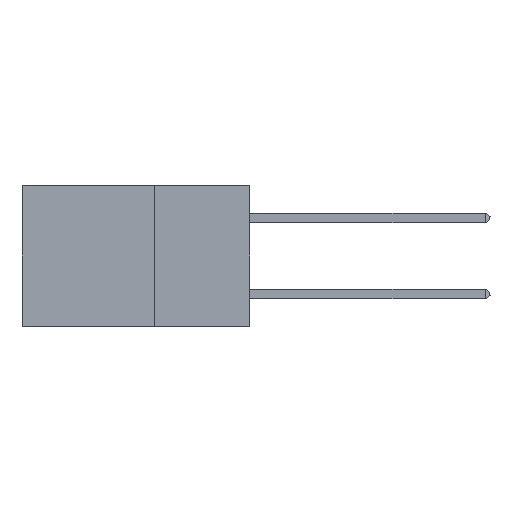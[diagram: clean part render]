
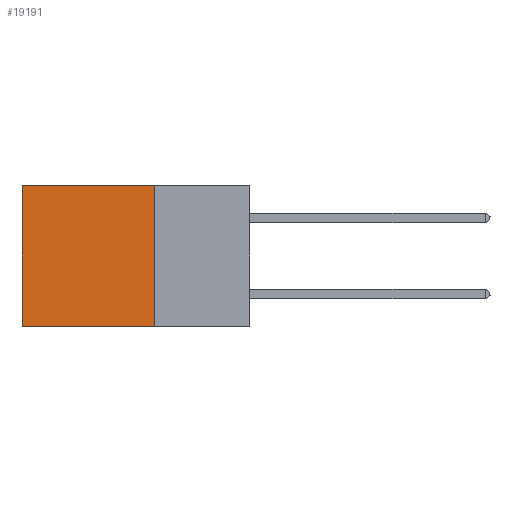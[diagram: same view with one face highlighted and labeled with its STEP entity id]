
A CAD part, left-side view. The second image highlights one B-rep face of the part: STEP entity #19191.
In plain terms, the highlighted planar face has unit normal (-1, 0, 0).
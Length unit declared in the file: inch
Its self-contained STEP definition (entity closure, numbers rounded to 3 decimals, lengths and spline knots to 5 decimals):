
#1883 = ORIENTED_EDGE ( 'NONE', *, *, #9768, .T. ) ;
#2938 = DIRECTION ( 'NONE',  ( 0., 1., 0. ) ) ;
#3231 = CARTESIAN_POINT ( 'NONE',  ( 0.2875, 0.25, -0.37 ) ) ;
#3572 = LINE ( 'NONE', #3231, #34149 ) ;
#4165 = LINE ( 'NONE', #35471, #8786 ) ;
#4431 = EDGE_LOOP ( 'NONE', ( #1883, #27763, #6067, #38843 ) ) ;
#4472 = CARTESIAN_POINT ( 'NONE',  ( 0.2875, 0.6, 0. ) ) ;
#6067 = ORIENTED_EDGE ( 'NONE', *, *, #7872, .F. ) ;
#7531 = LINE ( 'NONE', #43068, #9848 ) ;
#7872 = EDGE_CURVE ( 'NONE', #39668, #38257, #26251, .T. ) ;
#8786 = VECTOR ( 'NONE', #24356, 39.37008 ) ;
#9768 = EDGE_CURVE ( 'NONE', #15532, #27740, #4165, .T. ) ;
#9848 = VECTOR ( 'NONE', #2938, 39.37008 ) ;
#9864 = EDGE_CURVE ( 'NONE', #38257, #27740, #3572, .T. ) ;
#11196 = DIRECTION ( 'NONE',  ( 0., 0., -1. ) ) ;
#13850 = DIRECTION ( 'NONE',  ( 0., 1., 0. ) ) ;
#15532 = VERTEX_POINT ( 'NONE', #4472 ) ;
#15880 = CARTESIAN_POINT ( 'NONE',  ( 0.2875, 0.25, -0.37 ) ) ;
#19191 = ADVANCED_FACE ( 'NONE', ( #28418 ), #40385, .F. ) ;
#19772 = AXIS2_PLACEMENT_3D ( 'NONE', #40857, #47830, #11196 ) ;
#23465 = CARTESIAN_POINT ( 'NONE',  ( 0.2875, 0.25, 0. ) ) ;
#24356 = DIRECTION ( 'NONE',  ( 0., 0., -1. ) ) ;
#26251 = LINE ( 'NONE', #28870, #33779 ) ;
#27740 = VERTEX_POINT ( 'NONE', #31491 ) ;
#27763 = ORIENTED_EDGE ( 'NONE', *, *, #9864, .F. ) ;
#28418 = FACE_OUTER_BOUND ( 'NONE', #4431, .T. ) ;
#28870 = CARTESIAN_POINT ( 'NONE',  ( 0.2875, 0.25, 0. ) ) ;
#31491 = CARTESIAN_POINT ( 'NONE',  ( 0.2875, 0.6, -0.37 ) ) ;
#33779 = VECTOR ( 'NONE', #47294, 39.37008 ) ;
#34149 = VECTOR ( 'NONE', #13850, 39.37008 ) ;
#35471 = CARTESIAN_POINT ( 'NONE',  ( 0.2875, 0.6, 0. ) ) ;
#38257 = VERTEX_POINT ( 'NONE', #15880 ) ;
#38843 = ORIENTED_EDGE ( 'NONE', *, *, #45371, .T. ) ;
#39668 = VERTEX_POINT ( 'NONE', #23465 ) ;
#40385 = PLANE ( 'NONE',  #19772 ) ;
#40857 = CARTESIAN_POINT ( 'NONE',  ( 0.2875, 0.25, 0. ) ) ;
#43068 = CARTESIAN_POINT ( 'NONE',  ( 0.2875, 0.25, 0. ) ) ;
#45371 = EDGE_CURVE ( 'NONE', #39668, #15532, #7531, .T. ) ;
#47294 = DIRECTION ( 'NONE',  ( 0., 0., -1. ) ) ;
#47830 = DIRECTION ( 'NONE',  ( 1., 0., 0. ) ) ;
